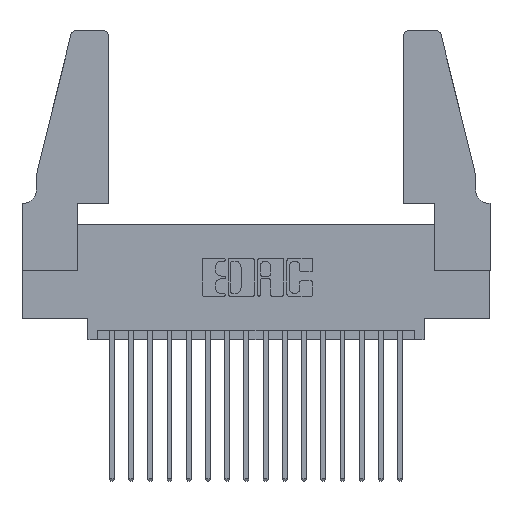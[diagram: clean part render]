
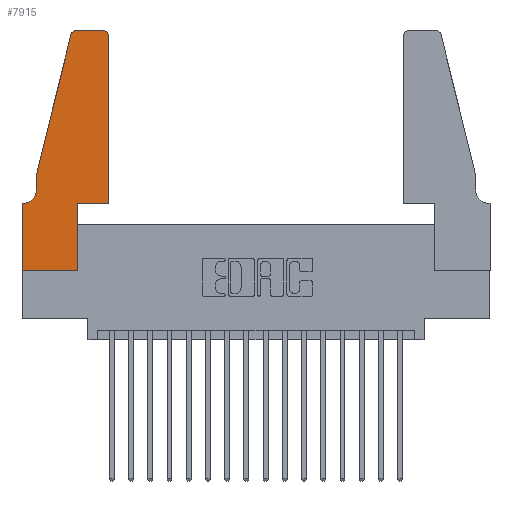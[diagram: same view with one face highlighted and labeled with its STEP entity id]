
A CAD part, top view. The second image highlights one B-rep face of the part: STEP entity #7915.
In plain terms, the highlighted planar face has unit normal (0, 0, 1).
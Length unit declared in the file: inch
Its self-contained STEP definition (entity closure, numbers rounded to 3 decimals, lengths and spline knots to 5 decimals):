
#208 = VECTOR ( 'NONE', #6945, 39.37008 ) ;
#292 = ORIENTED_EDGE ( 'NONE', *, *, #14328, .T. ) ;
#309 = ORIENTED_EDGE ( 'NONE', *, *, #7626, .T. ) ;
#315 = CARTESIAN_POINT ( 'NONE',  ( 0., 0.35, 0.37 ) ) ;
#537 = EDGE_CURVE ( 'NONE', #18008, #4355, #6023, .T. ) ;
#714 = VERTEX_POINT ( 'NONE', #13693 ) ;
#1013 = VERTEX_POINT ( 'NONE', #13239 ) ;
#1018 = VERTEX_POINT ( 'NONE', #14295 ) ;
#1070 = ORIENTED_EDGE ( 'NONE', *, *, #16928, .T. ) ;
#1204 = VERTEX_POINT ( 'NONE', #5243 ) ;
#2270 = ORIENTED_EDGE ( 'NONE', *, *, #10381, .T. ) ;
#2273 = AXIS2_PLACEMENT_3D ( 'NONE', #315, #16013, #7584 ) ;
#2328 = CARTESIAN_POINT ( 'NONE',  ( 0.2605, 1.25, 0.37 ) ) ;
#2333 = CARTESIAN_POINT ( 'NONE',  ( 0., 0., 0.37 ) ) ;
#2411 = EDGE_CURVE ( 'NONE', #13105, #15070, #10082, .T. ) ;
#2442 = CARTESIAN_POINT ( 'NONE',  ( 0., 0., 0.37 ) ) ;
#2672 = CARTESIAN_POINT ( 'NONE',  ( 0.0755, 0.35, 0.37 ) ) ;
#2718 = ORIENTED_EDGE ( 'NONE', *, *, #12814, .T. ) ;
#2898 = VECTOR ( 'NONE', #4070, 39.37008 ) ;
#3370 = PLANE ( 'NONE',  #2273 ) ;
#3377 = LINE ( 'NONE', #18056, #2898 ) ;
#3581 = VERTEX_POINT ( 'NONE', #13499 ) ;
#3803 = EDGE_CURVE ( 'NONE', #714, #9373, #10029, .T. ) ;
#3995 = CARTESIAN_POINT ( 'NONE',  ( 0.4205, 1.22, 0.37 ) ) ;
#4070 = DIRECTION ( 'NONE',  ( 0., 1., 0. ) ) ;
#4196 = LINE ( 'NONE', #2672, #208 ) ;
#4232 = EDGE_CURVE ( 'NONE', #14984, #1013, #17058, .T. ) ;
#4295 = CARTESIAN_POINT ( 'NONE',  ( 0., 0., 0.37 ) ) ;
#4355 = VERTEX_POINT ( 'NONE', #12440 ) ;
#4358 = CARTESIAN_POINT ( 'NONE',  ( 0.4505, 0.35, 0.37 ) ) ;
#4470 = EDGE_CURVE ( 'NONE', #15070, #1018, #5651, .T. ) ;
#4536 = DIRECTION ( 'NONE',  ( 0., 0., 1. ) ) ;
#4577 = EDGE_CURVE ( 'NONE', #1013, #16058, #11758, .T. ) ;
#4757 = CARTESIAN_POINT ( 'NONE',  ( 0.25487, 1.22718, 0.37 ) ) ;
#4935 = LINE ( 'NONE', #7109, #11490 ) ;
#5060 = CARTESIAN_POINT ( 'NONE',  ( 0.2865, 0.35, 0.37 ) ) ;
#5233 = DIRECTION ( 'NONE',  ( -1., 0., 0. ) ) ;
#5243 = CARTESIAN_POINT ( 'NONE',  ( 0.0055, 0.35, 0.37 ) ) ;
#5409 = DIRECTION ( 'NONE',  ( 1., 0., 0. ) ) ;
#5564 = AXIS2_PLACEMENT_3D ( 'NONE', #15596, #7178, #17015 ) ;
#5651 = LINE ( 'NONE', #4295, #9761 ) ;
#5701 = EDGE_CURVE ( 'NONE', #4355, #3581, #4935, .T. ) ;
#5875 = VECTOR ( 'NONE', #5233, 39.37008 ) ;
#6023 = LINE ( 'NONE', #4358, #9701 ) ;
#6248 = DIRECTION ( 'NONE',  ( 1., 0., 0. ) ) ;
#6709 = ORIENTED_EDGE ( 'NONE', *, *, #3803, .T. ) ;
#6945 = DIRECTION ( 'NONE',  ( -1., 0., 0. ) ) ;
#7034 = DIRECTION ( 'NONE',  ( 1., 0., 0. ) ) ;
#7109 = CARTESIAN_POINT ( 'NONE',  ( 0.4505, 0.35, 0.37 ) ) ;
#7178 = DIRECTION ( 'NONE',  ( 0., 0., -1. ) ) ;
#7254 = LINE ( 'NONE', #7752, #14307 ) ;
#7440 = DIRECTION ( 'NONE',  ( 0., -1., 0. ) ) ;
#7584 = DIRECTION ( 'NONE',  ( 1., 0., 0. ) ) ;
#7626 = EDGE_CURVE ( 'NONE', #1204, #13105, #4196, .T. ) ;
#7642 = DIRECTION ( 'NONE',  ( 0., -1., 0. ) ) ;
#7752 = CARTESIAN_POINT ( 'NONE',  ( 0.0755, 0.5, 0.37 ) ) ;
#7915 = ADVANCED_FACE ( 'NONE', ( #10956 ), #3370, .T. ) ;
#8252 = CARTESIAN_POINT ( 'NONE',  ( 0.0755, 0.5, 0.37 ) ) ;
#8712 = AXIS2_PLACEMENT_3D ( 'NONE', #12927, #4536, #14343 ) ;
#9065 = ORIENTED_EDGE ( 'NONE', *, *, #5701, .T. ) ;
#9261 = CARTESIAN_POINT ( 'NONE',  ( 0.4205, 1.25, 0.37 ) ) ;
#9373 = VERTEX_POINT ( 'NONE', #12094 ) ;
#9637 = VECTOR ( 'NONE', #7440, 39.37008 ) ;
#9701 = VECTOR ( 'NONE', #6248, 39.37008 ) ;
#9761 = VECTOR ( 'NONE', #7034, 39.37008 ) ;
#9998 = EDGE_LOOP ( 'NONE', ( #14632, #18315, #292, #6709, #2270, #309, #17585, #15058, #2718, #10845, #9065, #1070 ) ) ;
#10029 = LINE ( 'NONE', #8252, #16667 ) ;
#10082 = LINE ( 'NONE', #2333, #9637 ) ;
#10381 = EDGE_CURVE ( 'NONE', #9373, #1204, #16188, .T. ) ;
#10845 = ORIENTED_EDGE ( 'NONE', *, *, #537, .T. ) ;
#10956 = FACE_OUTER_BOUND ( 'NONE', #9998, .T. ) ;
#11490 = VECTOR ( 'NONE', #18240, 39.37008 ) ;
#11758 = CIRCLE ( 'NONE', #8712, 0.03 ) ;
#12094 = CARTESIAN_POINT ( 'NONE',  ( 0.0755, 0.42, 0.37 ) ) ;
#12440 = CARTESIAN_POINT ( 'NONE',  ( 0.4505, 0.35, 0.37 ) ) ;
#12814 = EDGE_CURVE ( 'NONE', #1018, #18008, #3377, .T. ) ;
#12927 = CARTESIAN_POINT ( 'NONE',  ( 0.284, 1.22, 0.37 ) ) ;
#13105 = VERTEX_POINT ( 'NONE', #16512 ) ;
#13239 = CARTESIAN_POINT ( 'NONE',  ( 0.284, 1.25, 0.37 ) ) ;
#13499 = CARTESIAN_POINT ( 'NONE',  ( 0.4505, 1.22, 0.37 ) ) ;
#13693 = CARTESIAN_POINT ( 'NONE',  ( 0.0755, 0.5, 0.37 ) ) ;
#13805 = DIRECTION ( 'NONE',  ( 0., 0., 1. ) ) ;
#14295 = CARTESIAN_POINT ( 'NONE',  ( 0.2865, 0., 0.37 ) ) ;
#14307 = VECTOR ( 'NONE', #14860, 39.37008 ) ;
#14328 = EDGE_CURVE ( 'NONE', #16058, #714, #7254, .T. ) ;
#14343 = DIRECTION ( 'NONE',  ( 1., 0., 0. ) ) ;
#14632 = ORIENTED_EDGE ( 'NONE', *, *, #4232, .T. ) ;
#14786 = AXIS2_PLACEMENT_3D ( 'NONE', #3995, #13805, #5409 ) ;
#14860 = DIRECTION ( 'NONE',  ( -0.239, -0.971, 0. ) ) ;
#14984 = VERTEX_POINT ( 'NONE', #9261 ) ;
#15058 = ORIENTED_EDGE ( 'NONE', *, *, #4470, .T. ) ;
#15070 = VERTEX_POINT ( 'NONE', #2442 ) ;
#15596 = CARTESIAN_POINT ( 'NONE',  ( 0.0055, 0.42, 0.37 ) ) ;
#16013 = DIRECTION ( 'NONE',  ( 0., 0., 1. ) ) ;
#16058 = VERTEX_POINT ( 'NONE', #4757 ) ;
#16188 = CIRCLE ( 'NONE', #5564, 0.07 ) ;
#16512 = CARTESIAN_POINT ( 'NONE',  ( 0., 0.35, 0.37 ) ) ;
#16667 = VECTOR ( 'NONE', #7642, 39.37008 ) ;
#16928 = EDGE_CURVE ( 'NONE', #3581, #14984, #18019, .T. ) ;
#17015 = DIRECTION ( 'NONE',  ( -1., 0., 0. ) ) ;
#17058 = LINE ( 'NONE', #2328, #5875 ) ;
#17585 = ORIENTED_EDGE ( 'NONE', *, *, #2411, .T. ) ;
#18008 = VERTEX_POINT ( 'NONE', #5060 ) ;
#18019 = CIRCLE ( 'NONE', #14786, 0.03 ) ;
#18056 = CARTESIAN_POINT ( 'NONE',  ( 0.2865, 0.35, 0.37 ) ) ;
#18240 = DIRECTION ( 'NONE',  ( 0., 1., 0. ) ) ;
#18315 = ORIENTED_EDGE ( 'NONE', *, *, #4577, .T. ) ;
